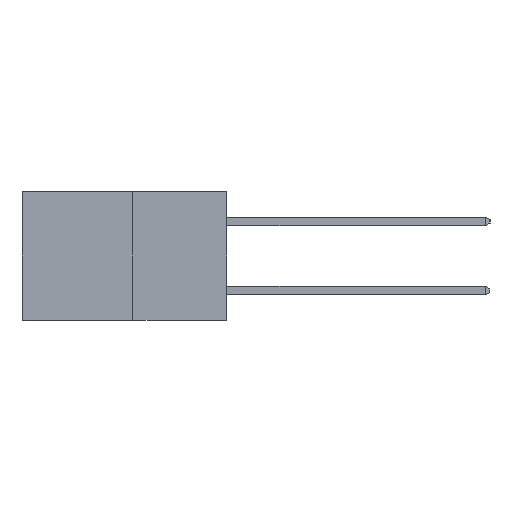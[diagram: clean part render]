
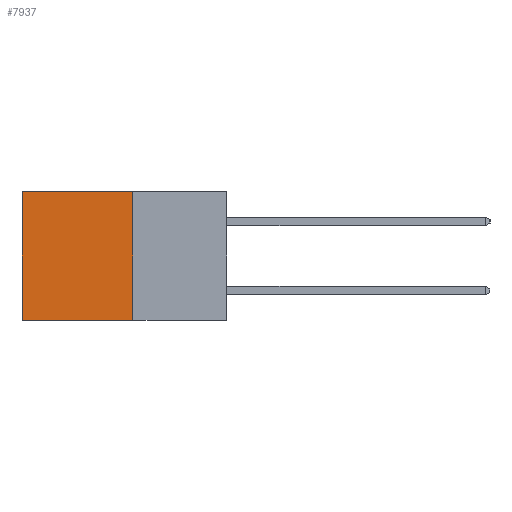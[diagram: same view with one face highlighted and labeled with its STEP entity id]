
A CAD part, left-side view. The second image highlights one B-rep face of the part: STEP entity #7937.
In plain terms, the highlighted planar face has unit normal (-1, 0, 0).
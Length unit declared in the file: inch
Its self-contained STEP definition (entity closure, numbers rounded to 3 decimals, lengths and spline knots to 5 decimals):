
#119 = VECTOR ( 'NONE', #3679, 39.37008 ) ;
#282 = DIRECTION ( 'NONE',  ( 0., 1., 0. ) ) ;
#468 = ORIENTED_EDGE ( 'NONE', *, *, #4674, .T. ) ;
#718 = CARTESIAN_POINT ( 'NONE',  ( 0.277, 0.27, -0.37 ) ) ;
#1490 = EDGE_LOOP ( 'NONE', ( #468, #11882, #6511, #10434 ) ) ;
#1681 = FACE_OUTER_BOUND ( 'NONE', #1490, .T. ) ;
#2299 = EDGE_CURVE ( 'NONE', #7211, #12424, #8435, .T. ) ;
#2406 = DIRECTION ( 'NONE',  ( 0., 1., 0. ) ) ;
#2771 = CARTESIAN_POINT ( 'NONE',  ( 0.277, 0.59, -0.37 ) ) ;
#2943 = EDGE_CURVE ( 'NONE', #12424, #5906, #5871, .T. ) ;
#3010 = VECTOR ( 'NONE', #282, 39.37008 ) ;
#3666 = CARTESIAN_POINT ( 'NONE',  ( 0.277, 0.27, -0.37 ) ) ;
#3679 = DIRECTION ( 'NONE',  ( 0., 0., -1. ) ) ;
#4002 = DIRECTION ( 'NONE',  ( 1., 0., 0. ) ) ;
#4674 = EDGE_CURVE ( 'NONE', #7270, #5906, #7190, .T. ) ;
#4891 = CARTESIAN_POINT ( 'NONE',  ( 0.277, 0.59, -0.37 ) ) ;
#5871 = LINE ( 'NONE', #11058, #3010 ) ;
#5906 = VERTEX_POINT ( 'NONE', #4891 ) ;
#6101 = LINE ( 'NONE', #11047, #11560 ) ;
#6421 = EDGE_CURVE ( 'NONE', #7211, #7270, #6101, .T. ) ;
#6511 = ORIENTED_EDGE ( 'NONE', *, *, #2299, .F. ) ;
#6960 = AXIS2_PLACEMENT_3D ( 'NONE', #718, #4002, #11600 ) ;
#7190 = LINE ( 'NONE', #2771, #7536 ) ;
#7211 = VERTEX_POINT ( 'NONE', #12310 ) ;
#7270 = VERTEX_POINT ( 'NONE', #8323 ) ;
#7536 = VECTOR ( 'NONE', #10357, 39.37008 ) ;
#7937 = ADVANCED_FACE ( 'NONE', ( #1681 ), #10528, .F. ) ;
#8323 = CARTESIAN_POINT ( 'NONE',  ( 0.277, 0.59, 0. ) ) ;
#8435 = LINE ( 'NONE', #3666, #119 ) ;
#10289 = CARTESIAN_POINT ( 'NONE',  ( 0.277, 0.27, -0.37 ) ) ;
#10357 = DIRECTION ( 'NONE',  ( 0., 0., -1. ) ) ;
#10434 = ORIENTED_EDGE ( 'NONE', *, *, #6421, .T. ) ;
#10528 = PLANE ( 'NONE',  #6960 ) ;
#11047 = CARTESIAN_POINT ( 'NONE',  ( 0.277, 0.27, 0. ) ) ;
#11058 = CARTESIAN_POINT ( 'NONE',  ( 0.277, 0.27, -0.37 ) ) ;
#11560 = VECTOR ( 'NONE', #2406, 39.37008 ) ;
#11600 = DIRECTION ( 'NONE',  ( 0., 0., -1. ) ) ;
#11882 = ORIENTED_EDGE ( 'NONE', *, *, #2943, .F. ) ;
#12310 = CARTESIAN_POINT ( 'NONE',  ( 0.277, 0.27, 0. ) ) ;
#12424 = VERTEX_POINT ( 'NONE', #10289 ) ;
